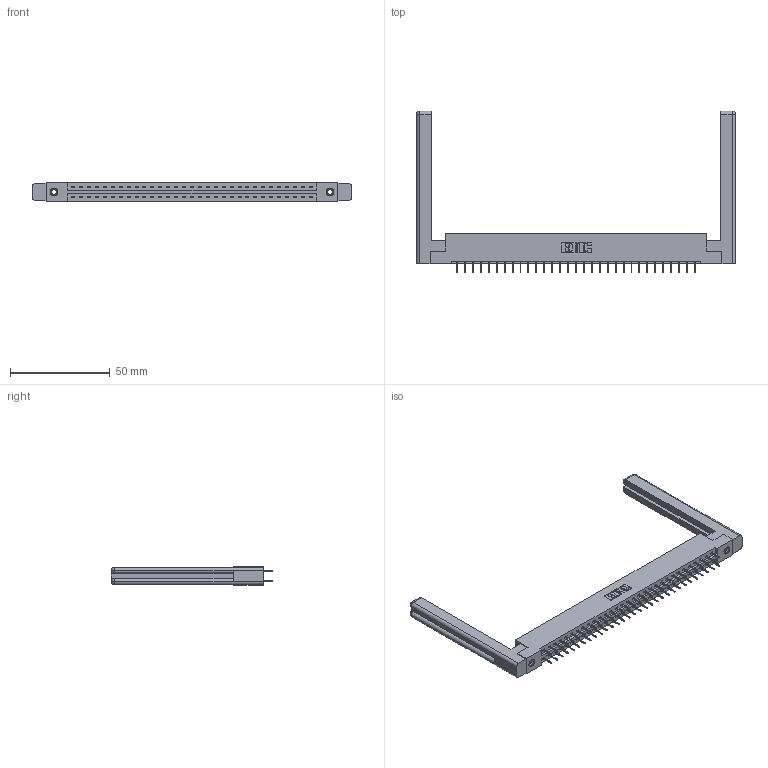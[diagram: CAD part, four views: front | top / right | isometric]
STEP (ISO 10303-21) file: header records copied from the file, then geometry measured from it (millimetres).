
FILE_DESCRIPTION (( 'STEP AP203' ), '1' );
FILE_NAME ('337-062-524-258.STEP', '2019-10-09T21:15:19', ( '' ), ( '' ), 'SwSTEP 2.0', 'SolidWorks 2016', '' );
FILE_SCHEMA (( 'CONFIG_CONTROL_DESIGN' ));
Length unit declared in the file: inch
Products named in the file (5): 337 Part_Flush Mounting Lugs - 0.156 Dia-TI; 337-062-524-258; 345-250-001_345-250-001-102; 345-292-001_345-293-124; 307-220-058
Assembly tree (67 placements, depth 2):
  337-062-524-258
    337 Part_Flush Mounting Lugs - 0.156 Dia-TI
    345-292-001_345-293-124  x62
    345-250-001_345-250-001-102  x2
    307-220-058  x2
Bounding box: 159.46 x 80.78 x 9.4 mm (x, y, z)
Volume: 23707.4 mm3; surface area: 23376.1 mm2
Topology: 67 solids, 67 shells, 3852 faces, 10895 edges, 7002 vertices
Faces by surface type: plane 2882, cylinder 946, cone 12, torus 12
Entity records: 28166 total; most frequent: CARTESIAN_POINT 4761, ORIENTED_EDGE 4636, DIRECTION 4086, EDGE_CURVE 2318, VECTOR 2146, LINE 2146, VERTEX_POINT 1534, AXIS2_PLACEMENT_3D 970
